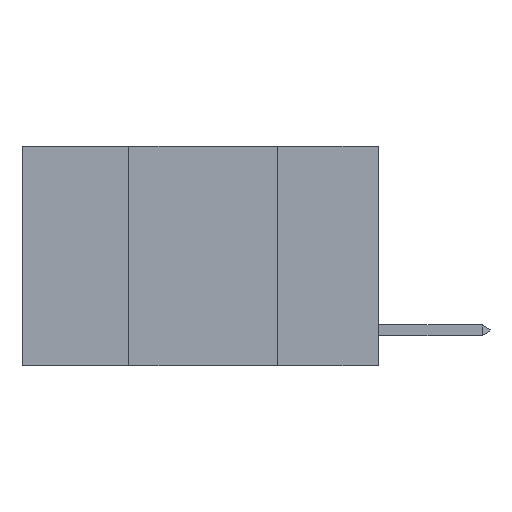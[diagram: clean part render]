
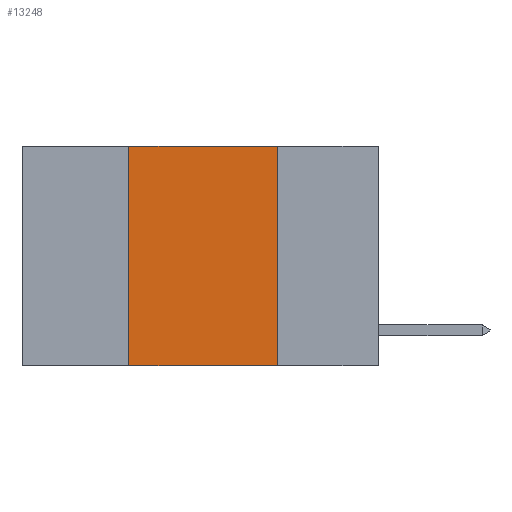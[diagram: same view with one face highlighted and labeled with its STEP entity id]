
A CAD part, left-side view. The second image highlights one B-rep face of the part: STEP entity #13248.
In plain terms, the highlighted planar face has unit normal (-1, 0, 0).
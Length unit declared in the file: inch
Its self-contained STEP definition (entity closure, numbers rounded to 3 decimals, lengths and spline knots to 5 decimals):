
#183 = ORIENTED_EDGE ( 'NONE', *, *, #4543, .F. ) ;
#2713 = AXIS2_PLACEMENT_3D ( 'NONE', #13346, #13407, #4885 ) ;
#4070 = VERTEX_POINT ( 'NONE', #11180 ) ;
#4543 = EDGE_CURVE ( 'NONE', #7835, #14104, #10250, .T. ) ;
#4885 = DIRECTION ( 'NONE',  ( 0., 0., -1. ) ) ;
#5593 = ORIENTED_EDGE ( 'NONE', *, *, #11693, .F. ) ;
#5756 = DIRECTION ( 'NONE',  ( 0., 0., -1. ) ) ;
#5930 = DIRECTION ( 'NONE',  ( 0., 0., 1. ) ) ;
#6498 = CARTESIAN_POINT ( 'NONE',  ( 0., 0.42, 0. ) ) ;
#7213 = VERTEX_POINT ( 'NONE', #9574 ) ;
#7835 = VERTEX_POINT ( 'NONE', #6498 ) ;
#8174 = EDGE_CURVE ( 'NONE', #14104, #4070, #16463, .T. ) ;
#9562 = CARTESIAN_POINT ( 'NONE',  ( 0., 0.17, 0. ) ) ;
#9574 = CARTESIAN_POINT ( 'NONE',  ( 0., 0.42, -0.37 ) ) ;
#9936 = CARTESIAN_POINT ( 'NONE',  ( 0., 0.17, 0. ) ) ;
#10207 = VECTOR ( 'NONE', #14828, 39.37008 ) ;
#10250 = LINE ( 'NONE', #15372, #13573 ) ;
#10518 = CARTESIAN_POINT ( 'NONE',  ( 0., 0.6, -0.37 ) ) ;
#10559 = VECTOR ( 'NONE', #5930, 39.37008 ) ;
#11180 = CARTESIAN_POINT ( 'NONE',  ( 0., 0.17, -0.37 ) ) ;
#11693 = EDGE_CURVE ( 'NONE', #7213, #7835, #13673, .T. ) ;
#13248 = ADVANCED_FACE ( 'NONE', ( #13629 ), #17510, .F. ) ;
#13346 = CARTESIAN_POINT ( 'NONE',  ( 0., 0.6, 0. ) ) ;
#13407 = DIRECTION ( 'NONE',  ( 1., 0., 0. ) ) ;
#13573 = VECTOR ( 'NONE', #14177, 39.37008 ) ;
#13629 = FACE_OUTER_BOUND ( 'NONE', #16488, .T. ) ;
#13673 = LINE ( 'NONE', #17114, #10559 ) ;
#14104 = VERTEX_POINT ( 'NONE', #9562 ) ;
#14177 = DIRECTION ( 'NONE',  ( 0., -1., 0. ) ) ;
#14467 = ORIENTED_EDGE ( 'NONE', *, *, #8174, .F. ) ;
#14504 = ORIENTED_EDGE ( 'NONE', *, *, #15171, .T. ) ;
#14828 = DIRECTION ( 'NONE',  ( 0., -1., 0. ) ) ;
#15171 = EDGE_CURVE ( 'NONE', #7213, #4070, #15468, .T. ) ;
#15372 = CARTESIAN_POINT ( 'NONE',  ( 0., 0.6, 0. ) ) ;
#15468 = LINE ( 'NONE', #10518, #10207 ) ;
#16463 = LINE ( 'NONE', #9936, #17370 ) ;
#16488 = EDGE_LOOP ( 'NONE', ( #14467, #183, #5593, #14504 ) ) ;
#17114 = CARTESIAN_POINT ( 'NONE',  ( 0., 0.42, 0. ) ) ;
#17370 = VECTOR ( 'NONE', #5756, 39.37008 ) ;
#17510 = PLANE ( 'NONE',  #2713 ) ;
